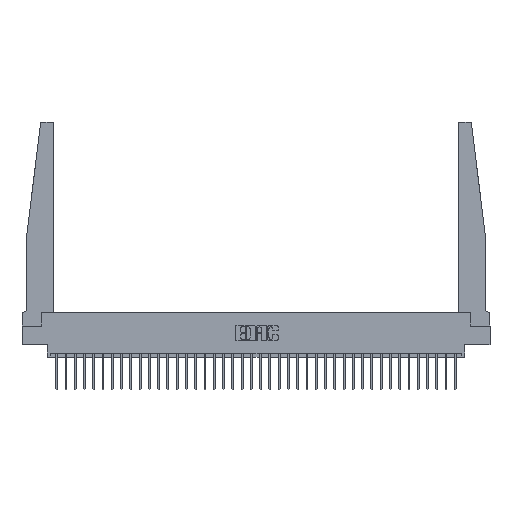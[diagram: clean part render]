
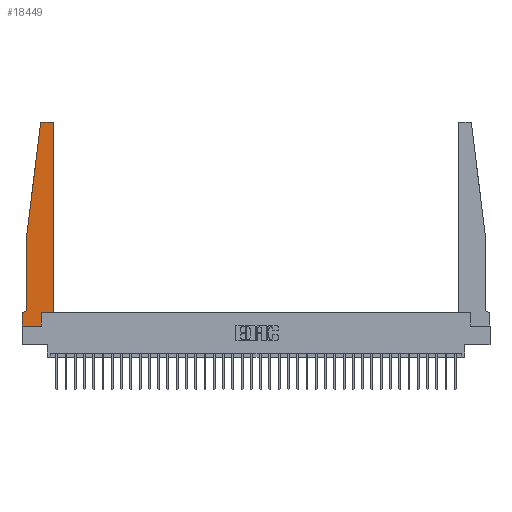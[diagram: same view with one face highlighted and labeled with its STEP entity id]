
A CAD part, top view. The second image highlights one B-rep face of the part: STEP entity #18449.
In plain terms, the highlighted planar face has unit normal (0, 0, 1).
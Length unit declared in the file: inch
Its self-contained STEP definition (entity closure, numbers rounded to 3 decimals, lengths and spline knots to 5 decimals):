
#39 = ORIENTED_EDGE ( 'NONE', *, *, #25289, .T. ) ;
#43 = ORIENTED_EDGE ( 'NONE', *, *, #3539, .T. ) ;
#63 = EDGE_CURVE ( 'NONE', #30689, #17186, #2150, .T. ) ;
#386 = VERTEX_POINT ( 'NONE', #25247 ) ;
#587 = ORIENTED_EDGE ( 'NONE', *, *, #11221, .T. ) ;
#1014 = EDGE_CURVE ( 'NONE', #26595, #386, #23508, .T. ) ;
#1806 = CIRCLE ( 'NONE', #23699, 0.03 ) ;
#2150 = LINE ( 'NONE', #15178, #29908 ) ;
#2991 = CARTESIAN_POINT ( 'NONE',  ( 0.065, 1.25, 0.37 ) ) ;
#3539 = EDGE_CURVE ( 'NONE', #20438, #21565, #9210, .T. ) ;
#4042 = VECTOR ( 'NONE', #5327, 39.37008 ) ;
#4335 = ORIENTED_EDGE ( 'NONE', *, *, #23445, .T. ) ;
#4609 = EDGE_CURVE ( 'NONE', #24242, #20438, #15260, .T. ) ;
#5203 = DIRECTION ( 'NONE',  ( 0., -1., 0. ) ) ;
#5327 = DIRECTION ( 'NONE',  ( 0., -1., 0. ) ) ;
#5530 = CIRCLE ( 'NONE', #19728, 0.03 ) ;
#5671 = CARTESIAN_POINT ( 'NONE',  ( 0., 0., 0.37 ) ) ;
#6138 = PLANE ( 'NONE',  #7322 ) ;
#6389 = DIRECTION ( 'NONE',  ( 0., 0., 1. ) ) ;
#6453 = CARTESIAN_POINT ( 'NONE',  ( 0.065, 0.2375, 0.37 ) ) ;
#6524 = VECTOR ( 'NONE', #21685, 39.37008 ) ;
#6570 = ORIENTED_EDGE ( 'NONE', *, *, #16637, .T. ) ;
#7045 = VECTOR ( 'NONE', #20965, 39.37008 ) ;
#7071 = VECTOR ( 'NONE', #18678, 39.37008 ) ;
#7205 = DIRECTION ( 'NONE',  ( 0., 1., 0. ) ) ;
#7322 = AXIS2_PLACEMENT_3D ( 'NONE', #27173, #13994, #11606 ) ;
#7777 = LINE ( 'NONE', #18232, #17615 ) ;
#8235 = LINE ( 'NONE', #32168, #7071 ) ;
#8357 = VECTOR ( 'NONE', #33580, 39.37008 ) ;
#8529 = ORIENTED_EDGE ( 'NONE', *, *, #63, .T. ) ;
#8696 = DIRECTION ( 'NONE',  ( -1., 0., 0. ) ) ;
#9055 = CARTESIAN_POINT ( 'NONE',  ( 0.065, 0.1875, 0.37 ) ) ;
#9200 = CARTESIAN_POINT ( 'NONE',  ( 0.015, 0.2375, 0.37 ) ) ;
#9210 = LINE ( 'NONE', #9055, #12862 ) ;
#9299 = ORIENTED_EDGE ( 'NONE', *, *, #16578, .T. ) ;
#9720 = DIRECTION ( 'NONE',  ( -1., 0., 0. ) ) ;
#10296 = VERTEX_POINT ( 'NONE', #13375 ) ;
#11221 = EDGE_CURVE ( 'NONE', #16299, #14770, #16212, .T. ) ;
#11606 = DIRECTION ( 'NONE',  ( 1., 0., 0. ) ) ;
#12017 = DIRECTION ( 'NONE',  ( 1., 0., 0. ) ) ;
#12862 = VECTOR ( 'NONE', #9720, 39.37008 ) ;
#13188 = CARTESIAN_POINT ( 'NONE',  ( 0.27653, 2.72, 0.37 ) ) ;
#13375 = CARTESIAN_POINT ( 'NONE',  ( 0.2605, 0.18, 0.37 ) ) ;
#13994 = DIRECTION ( 'NONE',  ( 0., 0., 1. ) ) ;
#14667 = FACE_OUTER_BOUND ( 'NONE', #21612, .T. ) ;
#14770 = VERTEX_POINT ( 'NONE', #2991 ) ;
#15178 = CARTESIAN_POINT ( 'NONE',  ( 0.25, 2.75, 0.37 ) ) ;
#15260 = CIRCLE ( 'NONE', #31118, 0.05 ) ;
#15424 = DIRECTION ( 'NONE',  ( 0., 0., 1. ) ) ;
#15994 = CARTESIAN_POINT ( 'NONE',  ( 0.395, 2.75, 0.37 ) ) ;
#16010 = CARTESIAN_POINT ( 'NONE',  ( 0.015, 0.1875, 0.37 ) ) ;
#16212 = LINE ( 'NONE', #26628, #6524 ) ;
#16299 = VERTEX_POINT ( 'NONE', #33135 ) ;
#16578 = EDGE_CURVE ( 'NONE', #10296, #27616, #30829, .T. ) ;
#16637 = EDGE_CURVE ( 'NONE', #27616, #22241, #25658, .T. ) ;
#17186 = VERTEX_POINT ( 'NONE', #32457 ) ;
#17603 = EDGE_CURVE ( 'NONE', #22241, #30689, #1806, .T. ) ;
#17615 = VECTOR ( 'NONE', #5203, 39.37008 ) ;
#18025 = ORIENTED_EDGE ( 'NONE', *, *, #1014, .T. ) ;
#18232 = CARTESIAN_POINT ( 'NONE',  ( 0.065, 1.25, 0.37 ) ) ;
#18352 = DIRECTION ( 'NONE',  ( 1., 0., 0. ) ) ;
#18449 = ADVANCED_FACE ( 'NONE', ( #14667 ), #6138, .T. ) ;
#18678 = DIRECTION ( 'NONE',  ( 0., 1., 0. ) ) ;
#19713 = ORIENTED_EDGE ( 'NONE', *, *, #29311, .T. ) ;
#19728 = AXIS2_PLACEMENT_3D ( 'NONE', #13188, #15424, #18352 ) ;
#19809 = ORIENTED_EDGE ( 'NONE', *, *, #4609, .T. ) ;
#20438 = VERTEX_POINT ( 'NONE', #16010 ) ;
#20916 = CARTESIAN_POINT ( 'NONE',  ( 0.425, 0.18, 0.37 ) ) ;
#20965 = DIRECTION ( 'NONE',  ( 1., 0., 0. ) ) ;
#21563 = CARTESIAN_POINT ( 'NONE',  ( 0.425, 0.18, 0.37 ) ) ;
#21565 = VERTEX_POINT ( 'NONE', #25188 ) ;
#21612 = EDGE_LOOP ( 'NONE', ( #8529, #4335, #587, #39, #19809, #43, #19713, #18025, #23603, #9299, #6570, #27265 ) ) ;
#21685 = DIRECTION ( 'NONE',  ( -0.122, -0.992, 0. ) ) ;
#21801 = CARTESIAN_POINT ( 'NONE',  ( 0.395, 2.72, 0.37 ) ) ;
#22219 = EDGE_CURVE ( 'NONE', #386, #10296, #8235, .T. ) ;
#22241 = VERTEX_POINT ( 'NONE', #29094 ) ;
#23228 = CARTESIAN_POINT ( 'NONE',  ( 0., 0., 0.37 ) ) ;
#23445 = EDGE_CURVE ( 'NONE', #17186, #16299, #5530, .T. ) ;
#23508 = LINE ( 'NONE', #31040, #7045 ) ;
#23603 = ORIENTED_EDGE ( 'NONE', *, *, #22219, .T. ) ;
#23642 = LINE ( 'NONE', #5671, #4042 ) ;
#23699 = AXIS2_PLACEMENT_3D ( 'NONE', #21801, #6389, #12017 ) ;
#23726 = DIRECTION ( 'NONE',  ( -1., 0., 0. ) ) ;
#24242 = VERTEX_POINT ( 'NONE', #6453 ) ;
#24417 = DIRECTION ( 'NONE',  ( 0., 0., -1. ) ) ;
#25188 = CARTESIAN_POINT ( 'NONE',  ( 0., 0.1875, 0.37 ) ) ;
#25247 = CARTESIAN_POINT ( 'NONE',  ( 0.2605, 0., 0.37 ) ) ;
#25254 = VECTOR ( 'NONE', #7205, 39.37008 ) ;
#25289 = EDGE_CURVE ( 'NONE', #14770, #24242, #7777, .T. ) ;
#25658 = LINE ( 'NONE', #28247, #25254 ) ;
#26595 = VERTEX_POINT ( 'NONE', #23228 ) ;
#26628 = CARTESIAN_POINT ( 'NONE',  ( 0.065, 1.25, 0.37 ) ) ;
#27173 = CARTESIAN_POINT ( 'NONE',  ( 0., 0.1875, 0.37 ) ) ;
#27265 = ORIENTED_EDGE ( 'NONE', *, *, #17603, .T. ) ;
#27616 = VERTEX_POINT ( 'NONE', #21563 ) ;
#28247 = CARTESIAN_POINT ( 'NONE',  ( 0.425, 0.18, 0.37 ) ) ;
#29094 = CARTESIAN_POINT ( 'NONE',  ( 0.425, 2.72, 0.37 ) ) ;
#29311 = EDGE_CURVE ( 'NONE', #21565, #26595, #23642, .T. ) ;
#29908 = VECTOR ( 'NONE', #23726, 39.37008 ) ;
#30689 = VERTEX_POINT ( 'NONE', #15994 ) ;
#30829 = LINE ( 'NONE', #20916, #8357 ) ;
#31040 = CARTESIAN_POINT ( 'NONE',  ( 0., 0., 0.37 ) ) ;
#31118 = AXIS2_PLACEMENT_3D ( 'NONE', #9200, #24417, #8696 ) ;
#32168 = CARTESIAN_POINT ( 'NONE',  ( 0.2605, 0.18, 0.37 ) ) ;
#32457 = CARTESIAN_POINT ( 'NONE',  ( 0.27653, 2.75, 0.37 ) ) ;
#33135 = CARTESIAN_POINT ( 'NONE',  ( 0.24675, 2.72367, 0.37 ) ) ;
#33580 = DIRECTION ( 'NONE',  ( 1., 0., 0. ) ) ;
